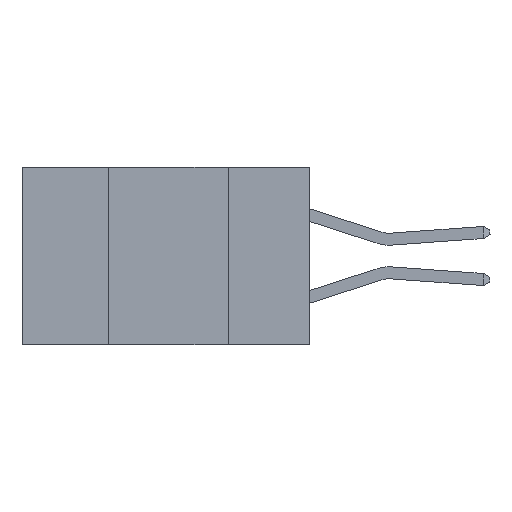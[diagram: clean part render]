
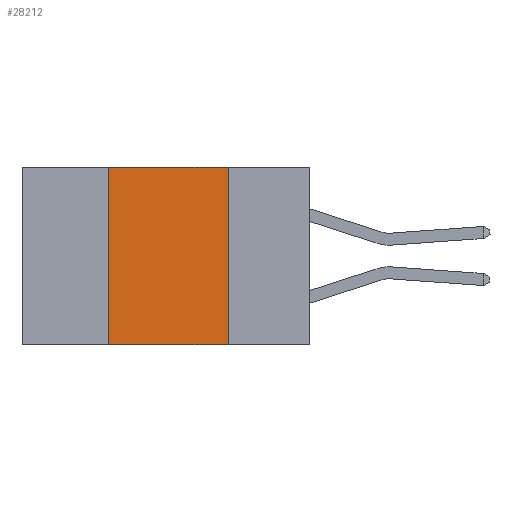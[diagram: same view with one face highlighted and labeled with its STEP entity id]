
A CAD part, left-side view. The second image highlights one B-rep face of the part: STEP entity #28212.
In plain terms, the highlighted planar face has unit normal (-1, 0, 0).
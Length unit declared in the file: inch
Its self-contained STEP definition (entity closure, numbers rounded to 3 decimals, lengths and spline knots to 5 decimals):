
#420 = VECTOR ( 'NONE', #8323, 39.37008 ) ;
#868 = PLANE ( 'NONE',  #10990 ) ;
#1463 = ORIENTED_EDGE ( 'NONE', *, *, #14432, .F. ) ;
#2343 = VECTOR ( 'NONE', #16528, 39.37008 ) ;
#3204 = DIRECTION ( 'NONE',  ( 0., 0., -1. ) ) ;
#4764 = VERTEX_POINT ( 'NONE', #19449 ) ;
#4980 = EDGE_CURVE ( 'NONE', #21529, #4764, #16428, .T. ) ;
#6079 = EDGE_LOOP ( 'NONE', ( #1463, #13533, #21625, #11288 ) ) ;
#8027 = VERTEX_POINT ( 'NONE', #22349 ) ;
#8323 = DIRECTION ( 'NONE',  ( 0., -1., 0. ) ) ;
#8865 = CARTESIAN_POINT ( 'NONE',  ( 0., 0.17, -0.37 ) ) ;
#10990 = AXIS2_PLACEMENT_3D ( 'NONE', #27529, #16660, #3204 ) ;
#11288 = ORIENTED_EDGE ( 'NONE', *, *, #26989, .T. ) ;
#11553 = CARTESIAN_POINT ( 'NONE',  ( 0., 0.17, 0. ) ) ;
#12477 = FACE_OUTER_BOUND ( 'NONE', #6079, .T. ) ;
#12507 = VERTEX_POINT ( 'NONE', #8865 ) ;
#13533 = ORIENTED_EDGE ( 'NONE', *, *, #4980, .F. ) ;
#13787 = DIRECTION ( 'NONE',  ( 0., 0., -1. ) ) ;
#14432 = EDGE_CURVE ( 'NONE', #4764, #12507, #17474, .T. ) ;
#16428 = LINE ( 'NONE', #17109, #2343 ) ;
#16528 = DIRECTION ( 'NONE',  ( 0., -1., 0. ) ) ;
#16568 = CARTESIAN_POINT ( 'NONE',  ( 0., 0.42, 0. ) ) ;
#16660 = DIRECTION ( 'NONE',  ( 1., 0., 0. ) ) ;
#17109 = CARTESIAN_POINT ( 'NONE',  ( 0., 0.6, 0. ) ) ;
#17162 = VECTOR ( 'NONE', #21897, 39.37008 ) ;
#17474 = LINE ( 'NONE', #11553, #22575 ) ;
#19449 = CARTESIAN_POINT ( 'NONE',  ( 0., 0.17, 0. ) ) ;
#19689 = CARTESIAN_POINT ( 'NONE',  ( 0., 0.42, 0. ) ) ;
#21529 = VERTEX_POINT ( 'NONE', #16568 ) ;
#21601 = CARTESIAN_POINT ( 'NONE',  ( 0., 0.6, -0.37 ) ) ;
#21625 = ORIENTED_EDGE ( 'NONE', *, *, #22458, .F. ) ;
#21897 = DIRECTION ( 'NONE',  ( 0., 0., 1. ) ) ;
#22349 = CARTESIAN_POINT ( 'NONE',  ( 0., 0.42, -0.37 ) ) ;
#22458 = EDGE_CURVE ( 'NONE', #8027, #21529, #22949, .T. ) ;
#22575 = VECTOR ( 'NONE', #13787, 39.37008 ) ;
#22835 = LINE ( 'NONE', #21601, #420 ) ;
#22949 = LINE ( 'NONE', #19689, #17162 ) ;
#26989 = EDGE_CURVE ( 'NONE', #8027, #12507, #22835, .T. ) ;
#27529 = CARTESIAN_POINT ( 'NONE',  ( 0., 0.6, 0. ) ) ;
#28212 = ADVANCED_FACE ( 'NONE', ( #12477 ), #868, .F. ) ;
